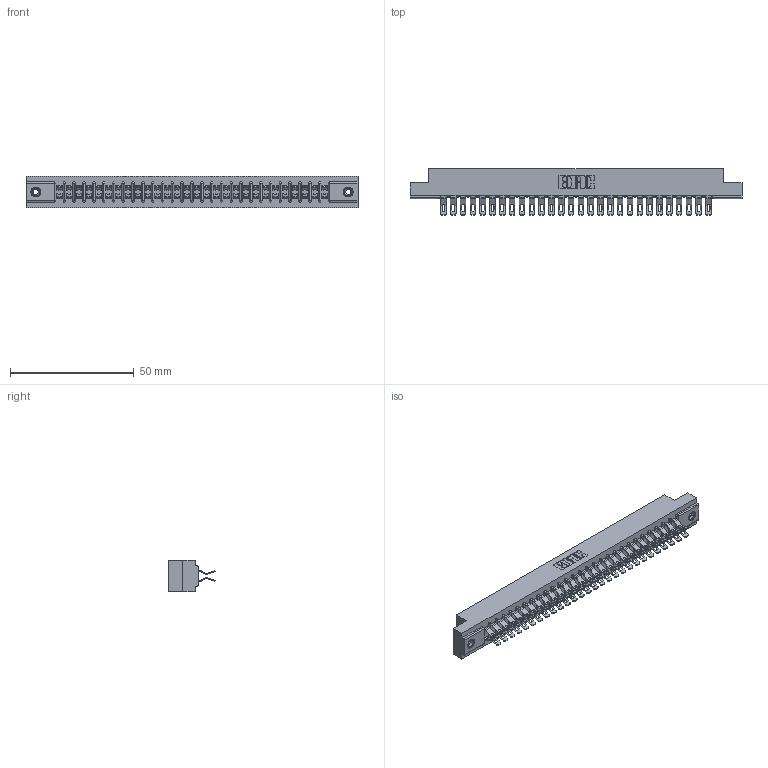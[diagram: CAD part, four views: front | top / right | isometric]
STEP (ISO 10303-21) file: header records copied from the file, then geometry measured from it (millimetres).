
FILE_DESCRIPTION (( 'STEP AP203' ), '1' );
FILE_NAME ('307-056-555-208.STEP', '2019-09-06T13:41:48', ( '' ), ( '' ), 'SwSTEP 2.0', 'SolidWorks 2016', '' );
FILE_SCHEMA (( 'CONFIG_CONTROL_DESIGN' ));
Length unit declared in the file: inch
Products named in the file (4): 345-250-001_345-250-003-102; 307-290-001_555; 307-056-555-208; 307 Part_.156 Dia Mounting Holes
Assembly tree (59 placements, depth 2):
  307-056-555-208
    307 Part_.156 Dia Mounting Holes
    307-290-001_555  x56
    345-250-001_345-250-003-102  x2
Bounding box: 133.96 x 18.75 x 12.7 mm (x, y, z)
Volume: 14306.1 mm3; surface area: 18168.5 mm2
Topology: 59 solids, 59 shells, 3623 faces, 10595 edges, 6902 vertices
Faces by surface type: plane 2006, cylinder 1543, sphere 58, cone 12, torus 4
Entity records: 28348 total; most frequent: CARTESIAN_POINT 4631, ORIENTED_EDGE 4584, DIRECTION 4558, EDGE_CURVE 2292, VECTOR 1740, LINE 1740, VERTEX_POINT 1482, AXIS2_PLACEMENT_3D 1409
